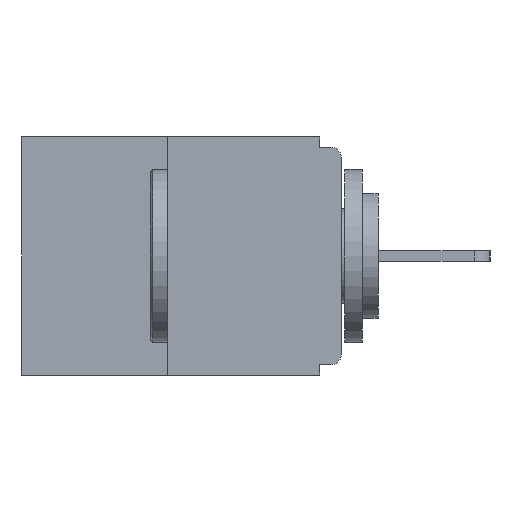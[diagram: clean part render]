
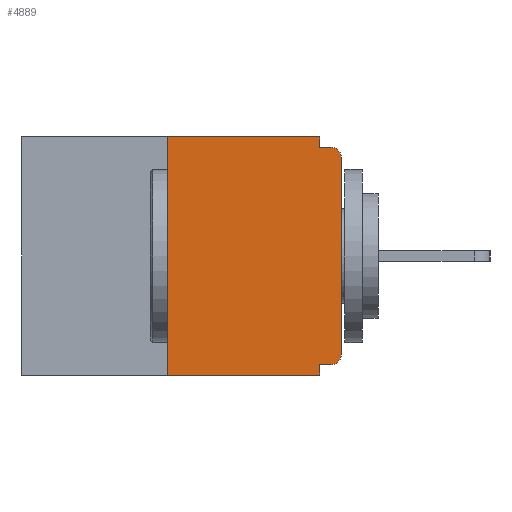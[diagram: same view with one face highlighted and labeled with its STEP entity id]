
A CAD part, left-side view. The second image highlights one B-rep face of the part: STEP entity #4889.
In plain terms, the highlighted planar face has unit normal (-1, 0, 0).
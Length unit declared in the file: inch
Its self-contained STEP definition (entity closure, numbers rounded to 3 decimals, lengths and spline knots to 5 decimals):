
#48 = CARTESIAN_POINT ( 'NONE',  ( 0., 0., -0.313 ) ) ;
#411 = EDGE_CURVE ( 'NONE', #16565, #16527, #19869, .T. ) ;
#512 = CARTESIAN_POINT ( 'NONE',  ( 0., 0.25, -0.343 ) ) ;
#758 = DIRECTION ( 'NONE',  ( 0., 0., -1. ) ) ;
#1152 = LINE ( 'NONE', #2989, #15602 ) ;
#1239 = VECTOR ( 'NONE', #6008, 39.37008 ) ;
#1624 = ORIENTED_EDGE ( 'NONE', *, *, #17564, .T. ) ;
#1741 = ORIENTED_EDGE ( 'NONE', *, *, #18713, .F. ) ;
#2169 = CARTESIAN_POINT ( 'NONE',  ( 0., 0.46, 0. ) ) ;
#2325 = VERTEX_POINT ( 'NONE', #3349 ) ;
#2554 = VECTOR ( 'NONE', #8766, 39.37008 ) ;
#2989 = CARTESIAN_POINT ( 'NONE',  ( 0., 0., -0.328 ) ) ;
#3170 = DIRECTION ( 'NONE',  ( 0., -1., 0. ) ) ;
#3349 = CARTESIAN_POINT ( 'NONE',  ( 0., 0.25, 0. ) ) ;
#3365 = CARTESIAN_POINT ( 'NONE',  ( 0., 0.015, -0.015 ) ) ;
#3904 = PLANE ( 'NONE',  #5100 ) ;
#3992 = DIRECTION ( 'NONE',  ( -1., 0., 0. ) ) ;
#4565 = AXIS2_PLACEMENT_3D ( 'NONE', #15030, #5276, #11485 ) ;
#4889 = ADVANCED_FACE ( 'NONE', ( #14575 ), #3904, .F. ) ;
#5045 = ORIENTED_EDGE ( 'NONE', *, *, #411, .F. ) ;
#5100 = AXIS2_PLACEMENT_3D ( 'NONE', #2169, #11337, #12945 ) ;
#5276 = DIRECTION ( 'NONE',  ( -1., 0., 0. ) ) ;
#5819 = VERTEX_POINT ( 'NONE', #10062 ) ;
#6008 = DIRECTION ( 'NONE',  ( 0., 0., 1. ) ) ;
#6136 = ORIENTED_EDGE ( 'NONE', *, *, #18018, .F. ) ;
#6269 = CARTESIAN_POINT ( 'NONE',  ( 0., 0.031, -0.343 ) ) ;
#6425 = CARTESIAN_POINT ( 'NONE',  ( 0., 0.46, 0. ) ) ;
#6721 = CARTESIAN_POINT ( 'NONE',  ( 0., 0., -0.03 ) ) ;
#6754 = CARTESIAN_POINT ( 'NONE',  ( 0., 0.031, -0.328 ) ) ;
#6762 = EDGE_CURVE ( 'NONE', #18960, #14658, #18734, .T. ) ;
#6829 = VERTEX_POINT ( 'NONE', #6721 ) ;
#7124 = EDGE_LOOP ( 'NONE', ( #10176, #6136, #17381, #1741, #19820, #1624, #10302, #14443, #5045, #11213 ) ) ;
#7234 = EDGE_CURVE ( 'NONE', #17471, #16565, #16494, .T. ) ;
#7308 = EDGE_CURVE ( 'NONE', #15575, #6829, #18113, .T. ) ;
#7766 = CARTESIAN_POINT ( 'NONE',  ( 0., 0., -0.015 ) ) ;
#8317 = LINE ( 'NONE', #10135, #12958 ) ;
#8746 = VECTOR ( 'NONE', #12823, 39.37008 ) ;
#8766 = DIRECTION ( 'NONE',  ( 0., 0., -1. ) ) ;
#8857 = CARTESIAN_POINT ( 'NONE',  ( 0., 0.25, 0. ) ) ;
#9107 = DIRECTION ( 'NONE',  ( 0., 1., 0. ) ) ;
#10062 = CARTESIAN_POINT ( 'NONE',  ( 0., 0.015, -0.328 ) ) ;
#10135 = CARTESIAN_POINT ( 'NONE',  ( 0., 0.031, -0.343 ) ) ;
#10176 = ORIENTED_EDGE ( 'NONE', *, *, #14275, .F. ) ;
#10302 = ORIENTED_EDGE ( 'NONE', *, *, #7308, .T. ) ;
#10438 = EDGE_CURVE ( 'NONE', #5819, #15183, #1152, .T. ) ;
#10685 = DIRECTION ( 'NONE',  ( 0., 0., 1. ) ) ;
#10992 = CARTESIAN_POINT ( 'NONE',  ( 0., 0.46, -0.343 ) ) ;
#11038 = AXIS2_PLACEMENT_3D ( 'NONE', #11737, #3992, #14876 ) ;
#11213 = ORIENTED_EDGE ( 'NONE', *, *, #7234, .F. ) ;
#11337 = DIRECTION ( 'NONE',  ( 1., 0., 0. ) ) ;
#11485 = DIRECTION ( 'NONE',  ( 0., 0., -1. ) ) ;
#11737 = CARTESIAN_POINT ( 'NONE',  ( 0., 0.015, -0.313 ) ) ;
#11918 = CARTESIAN_POINT ( 'NONE',  ( 0., 0., 0. ) ) ;
#12669 = VECTOR ( 'NONE', #10685, 39.37008 ) ;
#12688 = CIRCLE ( 'NONE', #4565, 0.015 ) ;
#12823 = DIRECTION ( 'NONE',  ( 0., -1., 0. ) ) ;
#12915 = CARTESIAN_POINT ( 'NONE',  ( 0., 0.031, -0.015 ) ) ;
#12945 = DIRECTION ( 'NONE',  ( 0., 0., -1. ) ) ;
#12958 = VECTOR ( 'NONE', #758, 39.37008 ) ;
#13555 = CARTESIAN_POINT ( 'NONE',  ( 0., 0.031, 0. ) ) ;
#13633 = CARTESIAN_POINT ( 'NONE',  ( 0., 0.031, 0. ) ) ;
#14275 = EDGE_CURVE ( 'NONE', #2325, #17471, #19045, .T. ) ;
#14443 = ORIENTED_EDGE ( 'NONE', *, *, #20004, .T. ) ;
#14488 = VECTOR ( 'NONE', #3170, 39.37008 ) ;
#14575 = FACE_OUTER_BOUND ( 'NONE', #7124, .T. ) ;
#14658 = VERTEX_POINT ( 'NONE', #6269 ) ;
#14876 = DIRECTION ( 'NONE',  ( 0., 0., -1. ) ) ;
#15030 = CARTESIAN_POINT ( 'NONE',  ( 0., 0.015, -0.03 ) ) ;
#15183 = VERTEX_POINT ( 'NONE', #6754 ) ;
#15575 = VERTEX_POINT ( 'NONE', #48 ) ;
#15602 = VECTOR ( 'NONE', #9107, 39.37008 ) ;
#15690 = DIRECTION ( 'NONE',  ( 0., -1., 0. ) ) ;
#16494 = LINE ( 'NONE', #13633, #2554 ) ;
#16527 = VERTEX_POINT ( 'NONE', #3365 ) ;
#16565 = VERTEX_POINT ( 'NONE', #12915 ) ;
#17206 = CIRCLE ( 'NONE', #11038, 0.015 ) ;
#17381 = ORIENTED_EDGE ( 'NONE', *, *, #6762, .T. ) ;
#17386 = VECTOR ( 'NONE', #15690, 39.37008 ) ;
#17471 = VERTEX_POINT ( 'NONE', #13555 ) ;
#17564 = EDGE_CURVE ( 'NONE', #5819, #15575, #17206, .T. ) ;
#18018 = EDGE_CURVE ( 'NONE', #18960, #2325, #18416, .T. ) ;
#18113 = LINE ( 'NONE', #11918, #1239 ) ;
#18416 = LINE ( 'NONE', #8857, #12669 ) ;
#18713 = EDGE_CURVE ( 'NONE', #15183, #14658, #8317, .T. ) ;
#18734 = LINE ( 'NONE', #10992, #17386 ) ;
#18960 = VERTEX_POINT ( 'NONE', #512 ) ;
#19045 = LINE ( 'NONE', #6425, #8746 ) ;
#19820 = ORIENTED_EDGE ( 'NONE', *, *, #10438, .F. ) ;
#19869 = LINE ( 'NONE', #7766, #14488 ) ;
#20004 = EDGE_CURVE ( 'NONE', #6829, #16527, #12688, .T. ) ;
